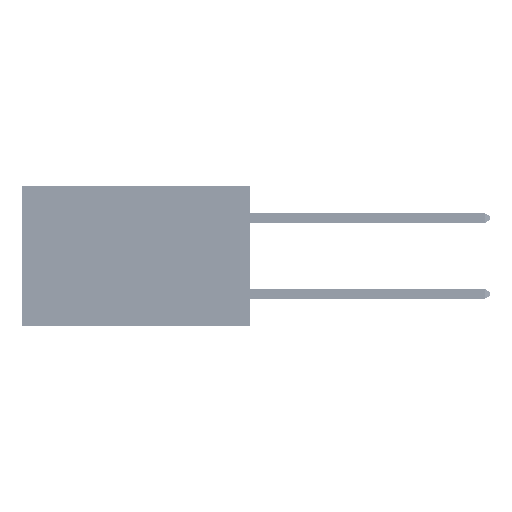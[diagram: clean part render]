
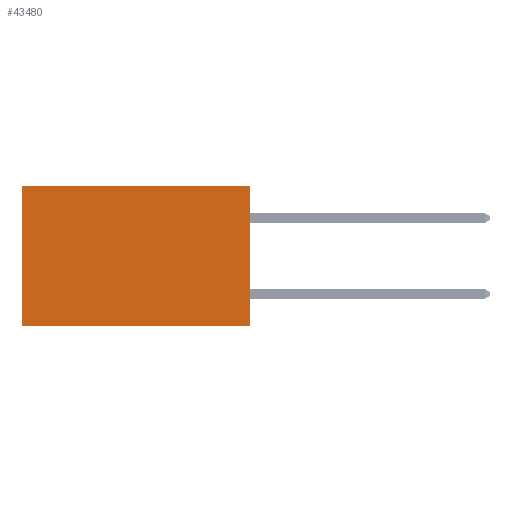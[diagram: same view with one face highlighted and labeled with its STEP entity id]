
A CAD part, left-side view. The second image highlights one B-rep face of the part: STEP entity #43480.
In plain terms, the highlighted planar face has unit normal (-1, 0, 0).
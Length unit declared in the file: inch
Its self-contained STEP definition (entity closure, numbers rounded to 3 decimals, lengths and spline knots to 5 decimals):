
#94 = CARTESIAN_POINT ( 'NONE',  ( 0.2875, 0.6, -0.37 ) ) ;
#2872 = CARTESIAN_POINT ( 'NONE',  ( 0.2875, 0.6, 0. ) ) ;
#7231 = CARTESIAN_POINT ( 'NONE',  ( 0.2875, 0., 0. ) ) ;
#7524 = EDGE_LOOP ( 'NONE', ( #9307, #44267, #41313, #19903 ) ) ;
#9307 = ORIENTED_EDGE ( 'NONE', *, *, #32302, .T. ) ;
#11987 = LINE ( 'NONE', #18055, #31251 ) ;
#14953 = DIRECTION ( 'NONE',  ( 1., 0., 0. ) ) ;
#15342 = VECTOR ( 'NONE', #40330, 39.37008 ) ;
#18055 = CARTESIAN_POINT ( 'NONE',  ( 0.2875, 0., 0. ) ) ;
#19903 = ORIENTED_EDGE ( 'NONE', *, *, #35108, .T. ) ;
#22979 = CARTESIAN_POINT ( 'NONE',  ( 0.2875, 0., -0.37 ) ) ;
#23219 = VECTOR ( 'NONE', #29869, 39.37008 ) ;
#23764 = EDGE_CURVE ( 'NONE', #30937, #23857, #45597, .T. ) ;
#23857 = VERTEX_POINT ( 'NONE', #94 ) ;
#29869 = DIRECTION ( 'NONE',  ( 0., 0., -1. ) ) ;
#30537 = CARTESIAN_POINT ( 'NONE',  ( 0.2875, 0., -0.37 ) ) ;
#30937 = VERTEX_POINT ( 'NONE', #22979 ) ;
#31251 = VECTOR ( 'NONE', #48516, 39.37008 ) ;
#32226 = LINE ( 'NONE', #2872, #23219 ) ;
#32302 = EDGE_CURVE ( 'NONE', #35776, #23857, #32226, .T. ) ;
#33288 = CARTESIAN_POINT ( 'NONE',  ( 0.2875, 0.6, 0. ) ) ;
#33653 = VERTEX_POINT ( 'NONE', #41345 ) ;
#34321 = DIRECTION ( 'NONE',  ( 0., 1., 0. ) ) ;
#35108 = EDGE_CURVE ( 'NONE', #33653, #35776, #48169, .T. ) ;
#35549 = VECTOR ( 'NONE', #34321, 39.37008 ) ;
#35776 = VERTEX_POINT ( 'NONE', #33288 ) ;
#36507 = CARTESIAN_POINT ( 'NONE',  ( 0.2875, 0., 0. ) ) ;
#38559 = EDGE_CURVE ( 'NONE', #33653, #30937, #11987, .T. ) ;
#40330 = DIRECTION ( 'NONE',  ( 0., 1., 0. ) ) ;
#41313 = ORIENTED_EDGE ( 'NONE', *, *, #38559, .F. ) ;
#41345 = CARTESIAN_POINT ( 'NONE',  ( 0.2875, 0., 0. ) ) ;
#41738 = DIRECTION ( 'NONE',  ( 0., 0., -1. ) ) ;
#43480 = ADVANCED_FACE ( 'NONE', ( #45349 ), #49137, .F. ) ;
#44267 = ORIENTED_EDGE ( 'NONE', *, *, #23764, .F. ) ;
#44422 = AXIS2_PLACEMENT_3D ( 'NONE', #7231, #14953, #41738 ) ;
#45349 = FACE_OUTER_BOUND ( 'NONE', #7524, .T. ) ;
#45597 = LINE ( 'NONE', #30537, #35549 ) ;
#48169 = LINE ( 'NONE', #36507, #15342 ) ;
#48516 = DIRECTION ( 'NONE',  ( 0., 0., -1. ) ) ;
#49137 = PLANE ( 'NONE',  #44422 ) ;
